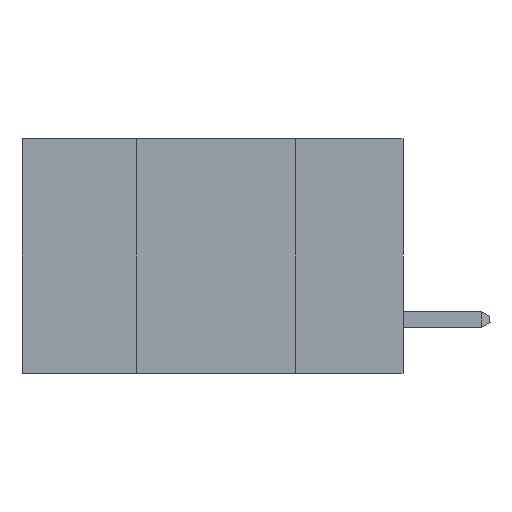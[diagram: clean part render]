
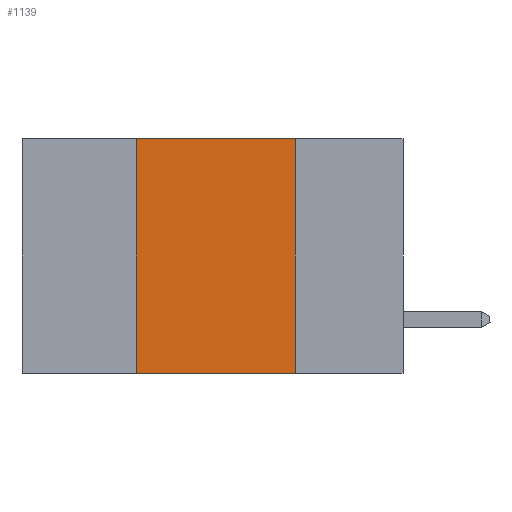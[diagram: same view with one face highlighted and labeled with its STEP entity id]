
A CAD part, left-side view. The second image highlights one B-rep face of the part: STEP entity #1139.
In plain terms, the highlighted planar face has unit normal (-1, 0, 0).
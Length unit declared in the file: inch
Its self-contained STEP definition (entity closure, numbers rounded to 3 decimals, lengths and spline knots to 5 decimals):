
#179 = CARTESIAN_POINT ( 'NONE',  ( 0., 0.6, 0. ) ) ;
#478 = ORIENTED_EDGE ( 'NONE', *, *, #30109, .F. ) ;
#1139 = ADVANCED_FACE ( 'NONE', ( #8415 ), #7310, .F. ) ;
#2280 = VECTOR ( 'NONE', #40224, 39.37008 ) ;
#3114 = VERTEX_POINT ( 'NONE', #7399 ) ;
#7310 = PLANE ( 'NONE',  #36722 ) ;
#7399 = CARTESIAN_POINT ( 'NONE',  ( 0., 0.17, -0.37 ) ) ;
#8415 = FACE_OUTER_BOUND ( 'NONE', #38418, .T. ) ;
#8443 = LINE ( 'NONE', #10304, #12025 ) ;
#9821 = CARTESIAN_POINT ( 'NONE',  ( 0., 0.17, 0. ) ) ;
#10304 = CARTESIAN_POINT ( 'NONE',  ( 0., 0.42, 0. ) ) ;
#12025 = VECTOR ( 'NONE', #43877, 39.37008 ) ;
#15370 = DIRECTION ( 'NONE',  ( 0., 0., -1. ) ) ;
#16198 = LINE ( 'NONE', #9821, #18619 ) ;
#17965 = ORIENTED_EDGE ( 'NONE', *, *, #31513, .F. ) ;
#18619 = VECTOR ( 'NONE', #43364, 39.37008 ) ;
#18814 = DIRECTION ( 'NONE',  ( 1., 0., 0. ) ) ;
#19179 = LINE ( 'NONE', #42363, #26913 ) ;
#21156 = LINE ( 'NONE', #38668, #2280 ) ;
#22370 = CARTESIAN_POINT ( 'NONE',  ( 0., 0.42, -0.37 ) ) ;
#24772 = CARTESIAN_POINT ( 'NONE',  ( 0., 0.17, 0. ) ) ;
#26913 = VECTOR ( 'NONE', #35068, 39.37008 ) ;
#29847 = EDGE_CURVE ( 'NONE', #43631, #3114, #19179, .T. ) ;
#30109 = EDGE_CURVE ( 'NONE', #39018, #44678, #21156, .T. ) ;
#31513 = EDGE_CURVE ( 'NONE', #44678, #3114, #16198, .T. ) ;
#32226 = CARTESIAN_POINT ( 'NONE',  ( 0., 0.42, 0. ) ) ;
#32904 = EDGE_CURVE ( 'NONE', #43631, #39018, #8443, .T. ) ;
#33333 = ORIENTED_EDGE ( 'NONE', *, *, #32904, .F. ) ;
#35068 = DIRECTION ( 'NONE',  ( 0., -1., 0. ) ) ;
#36722 = AXIS2_PLACEMENT_3D ( 'NONE', #179, #18814, #15370 ) ;
#38418 = EDGE_LOOP ( 'NONE', ( #17965, #478, #33333, #39158 ) ) ;
#38668 = CARTESIAN_POINT ( 'NONE',  ( 0., 0.6, 0. ) ) ;
#39018 = VERTEX_POINT ( 'NONE', #32226 ) ;
#39158 = ORIENTED_EDGE ( 'NONE', *, *, #29847, .T. ) ;
#40224 = DIRECTION ( 'NONE',  ( 0., -1., 0. ) ) ;
#42363 = CARTESIAN_POINT ( 'NONE',  ( 0., 0.6, -0.37 ) ) ;
#43364 = DIRECTION ( 'NONE',  ( 0., 0., -1. ) ) ;
#43631 = VERTEX_POINT ( 'NONE', #22370 ) ;
#43877 = DIRECTION ( 'NONE',  ( 0., 0., 1. ) ) ;
#44678 = VERTEX_POINT ( 'NONE', #24772 ) ;
